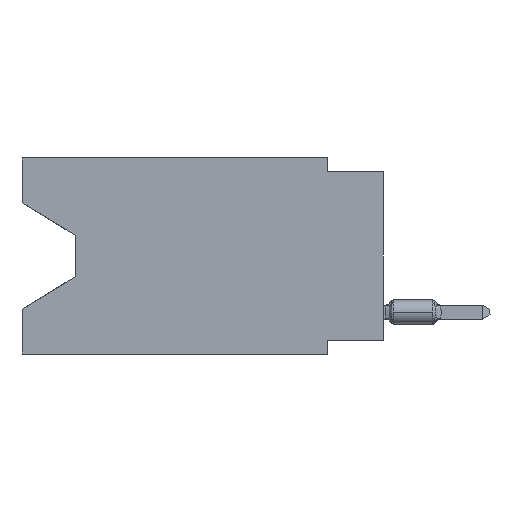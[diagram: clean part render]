
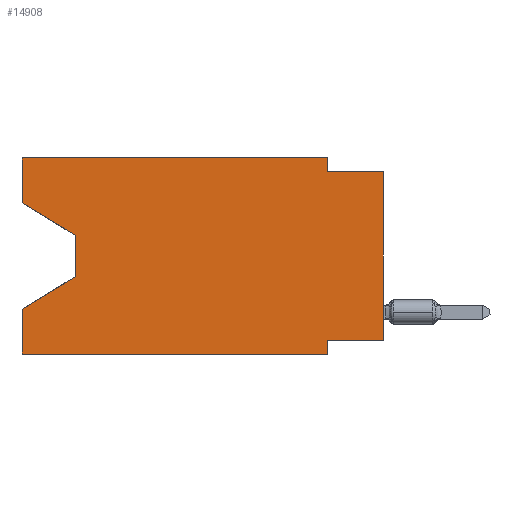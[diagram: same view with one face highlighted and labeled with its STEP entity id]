
A CAD part, left-side view. The second image highlights one B-rep face of the part: STEP entity #14908.
In plain terms, the highlighted planar face has unit normal (-1, 0, 0).
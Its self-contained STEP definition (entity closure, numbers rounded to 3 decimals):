
#5 = CARTESIAN_POINT ( 'NONE',  ( 0., 16.383, -8.89 ) ) ;
#255 = DIRECTION ( 'NONE',  ( 0., -1., 0. ) ) ;
#347 = VERTEX_POINT ( 'NONE', #15128 ) ;
#848 = LINE ( 'NONE', #18604, #24250 ) ;
#1271 = DIRECTION ( 'NONE',  ( 0., -1., 0. ) ) ;
#1398 = CARTESIAN_POINT ( 'NONE',  ( 0., 16.383, 0. ) ) ;
#1556 = CARTESIAN_POINT ( 'NONE',  ( 0., 13.97, -5.385 ) ) ;
#2352 = VERTEX_POINT ( 'NONE', #7971 ) ;
#2392 = VECTOR ( 'NONE', #1271, 1000. ) ;
#2432 = ORIENTED_EDGE ( 'NONE', *, *, #12009, .F. ) ;
#2817 = DIRECTION ( 'NONE',  ( 0., 1., 0. ) ) ;
#3191 = CARTESIAN_POINT ( 'NONE',  ( 0., 13.97, -3.505 ) ) ;
#3424 = EDGE_CURVE ( 'NONE', #2352, #17544, #19180, .T. ) ;
#3580 = VECTOR ( 'NONE', #3627, 1000. ) ;
#3627 = DIRECTION ( 'NONE',  ( 0., 0., 1. ) ) ;
#3709 = CARTESIAN_POINT ( 'NONE',  ( 0., 16.383, -2.038 ) ) ;
#4461 = VECTOR ( 'NONE', #10845, 1000. ) ;
#4632 = ORIENTED_EDGE ( 'NONE', *, *, #6374, .F. ) ;
#4938 = EDGE_CURVE ( 'NONE', #18866, #10406, #14768, .T. ) ;
#4984 = DIRECTION ( 'NONE',  ( 0., 0., 1. ) ) ;
#5467 = DIRECTION ( 'NONE',  ( 0., 0., -1. ) ) ;
#5589 = LINE ( 'NONE', #13303, #7961 ) ;
#5597 = VECTOR ( 'NONE', #24941, 1000. ) ;
#5640 = CARTESIAN_POINT ( 'NONE',  ( 0., 2.54, -8.89 ) ) ;
#5714 = DIRECTION ( 'NONE',  ( 0., -0.855, -0.519 ) ) ;
#5738 = CARTESIAN_POINT ( 'NONE',  ( 0., 16.383, 0. ) ) ;
#6042 = VERTEX_POINT ( 'NONE', #5640 ) ;
#6374 = EDGE_CURVE ( 'NONE', #17475, #347, #20489, .T. ) ;
#7307 = DIRECTION ( 'NONE',  ( 0., 0., -1. ) ) ;
#7353 = CARTESIAN_POINT ( 'NONE',  ( 0., 0., -0.635 ) ) ;
#7961 = VECTOR ( 'NONE', #5467, 1000. ) ;
#7971 = CARTESIAN_POINT ( 'NONE',  ( 0., 13.97, -5.385 ) ) ;
#8247 = VECTOR ( 'NONE', #255, 1000. ) ;
#8417 = FACE_OUTER_BOUND ( 'NONE', #22489, .T. ) ;
#8743 = CARTESIAN_POINT ( 'NONE',  ( 0., 13.97, -3.505 ) ) ;
#8981 = CARTESIAN_POINT ( 'NONE',  ( 0., 2.54, 0. ) ) ;
#9405 = EDGE_CURVE ( 'NONE', #24299, #10406, #15676, .T. ) ;
#9772 = ORIENTED_EDGE ( 'NONE', *, *, #4938, .F. ) ;
#10406 = VERTEX_POINT ( 'NONE', #7353 ) ;
#10473 = DIRECTION ( 'NONE',  ( 0., 0., -1. ) ) ;
#10730 = EDGE_CURVE ( 'NONE', #24299, #14086, #20434, .T. ) ;
#10845 = DIRECTION ( 'NONE',  ( 0., -1., 0. ) ) ;
#11954 = ORIENTED_EDGE ( 'NONE', *, *, #15281, .T. ) ;
#12009 = EDGE_CURVE ( 'NONE', #20213, #17544, #19030, .T. ) ;
#12262 = EDGE_CURVE ( 'NONE', #25340, #17475, #848, .T. ) ;
#12410 = VECTOR ( 'NONE', #25116, 1000. ) ;
#13276 = ORIENTED_EDGE ( 'NONE', *, *, #3424, .T. ) ;
#13303 = CARTESIAN_POINT ( 'NONE',  ( 0., 2.54, -8.89 ) ) ;
#13310 = VECTOR ( 'NONE', #5714, 1000. ) ;
#13683 = EDGE_CURVE ( 'NONE', #15964, #2352, #17064, .T. ) ;
#14086 = VERTEX_POINT ( 'NONE', #15706 ) ;
#14324 = PLANE ( 'NONE',  #23954 ) ;
#14700 = ORIENTED_EDGE ( 'NONE', *, *, #12262, .F. ) ;
#14768 = LINE ( 'NONE', #19029, #2392 ) ;
#14908 = ADVANCED_FACE ( 'NONE', ( #8417 ), #14324, .F. ) ;
#15128 = CARTESIAN_POINT ( 'NONE',  ( 0., 2.54, 0. ) ) ;
#15230 = EDGE_CURVE ( 'NONE', #14086, #6042, #5589, .T. ) ;
#15268 = LINE ( 'NONE', #8981, #5597 ) ;
#15281 = EDGE_CURVE ( 'NONE', #25340, #15964, #15470, .T. ) ;
#15470 = LINE ( 'NONE', #23341, #13310 ) ;
#15533 = DIRECTION ( 'NONE',  ( 0., 0., 1. ) ) ;
#15607 = VECTOR ( 'NONE', #15533, 1000. ) ;
#15676 = LINE ( 'NONE', #19803, #3580 ) ;
#15706 = CARTESIAN_POINT ( 'NONE',  ( 0., 2.54, -8.255 ) ) ;
#15964 = VERTEX_POINT ( 'NONE', #8743 ) ;
#16477 = VECTOR ( 'NONE', #2817, 1000. ) ;
#16571 = ORIENTED_EDGE ( 'NONE', *, *, #18057, .F. ) ;
#17064 = LINE ( 'NONE', #3191, #24024 ) ;
#17475 = VERTEX_POINT ( 'NONE', #5738 ) ;
#17544 = VERTEX_POINT ( 'NONE', #21934 ) ;
#17572 = ORIENTED_EDGE ( 'NONE', *, *, #13683, .T. ) ;
#18057 = EDGE_CURVE ( 'NONE', #347, #18866, #15268, .T. ) ;
#18187 = DIRECTION ( 'NONE',  ( 1., 0., 0. ) ) ;
#18604 = CARTESIAN_POINT ( 'NONE',  ( 0., 16.383, 0. ) ) ;
#18866 = VERTEX_POINT ( 'NONE', #20488 ) ;
#19029 = CARTESIAN_POINT ( 'NONE',  ( 0., 0., -0.635 ) ) ;
#19030 = LINE ( 'NONE', #1398, #15607 ) ;
#19180 = LINE ( 'NONE', #1556, #12410 ) ;
#19466 = LINE ( 'NONE', #25264, #8247 ) ;
#19803 = CARTESIAN_POINT ( 'NONE',  ( 0., 0., 0. ) ) ;
#20213 = VERTEX_POINT ( 'NONE', #5 ) ;
#20434 = LINE ( 'NONE', #20698, #16477 ) ;
#20488 = CARTESIAN_POINT ( 'NONE',  ( 0., 2.54, -0.635 ) ) ;
#20489 = LINE ( 'NONE', #20753, #4461 ) ;
#20698 = CARTESIAN_POINT ( 'NONE',  ( 0., 0., -8.255 ) ) ;
#20753 = CARTESIAN_POINT ( 'NONE',  ( 0., 16.383, 0. ) ) ;
#20826 = CARTESIAN_POINT ( 'NONE',  ( 0., 0., -8.255 ) ) ;
#21405 = EDGE_CURVE ( 'NONE', #20213, #6042, #19466, .T. ) ;
#21700 = ORIENTED_EDGE ( 'NONE', *, *, #9405, .T. ) ;
#21934 = CARTESIAN_POINT ( 'NONE',  ( 0., 16.383, -6.852 ) ) ;
#22489 = EDGE_LOOP ( 'NONE', ( #11954, #17572, #13276, #2432, #24428, #23222, #23672, #21700, #9772, #16571, #4632, #14700 ) ) ;
#23222 = ORIENTED_EDGE ( 'NONE', *, *, #15230, .F. ) ;
#23341 = CARTESIAN_POINT ( 'NONE',  ( 0., 16.383, -2.038 ) ) ;
#23672 = ORIENTED_EDGE ( 'NONE', *, *, #10730, .F. ) ;
#23954 = AXIS2_PLACEMENT_3D ( 'NONE', #24113, #18187, #10473 ) ;
#24024 = VECTOR ( 'NONE', #7307, 1000. ) ;
#24113 = CARTESIAN_POINT ( 'NONE',  ( 0., 16.383, 0. ) ) ;
#24250 = VECTOR ( 'NONE', #4984, 1000. ) ;
#24299 = VERTEX_POINT ( 'NONE', #20826 ) ;
#24428 = ORIENTED_EDGE ( 'NONE', *, *, #21405, .T. ) ;
#24941 = DIRECTION ( 'NONE',  ( 0., 0., -1. ) ) ;
#25116 = DIRECTION ( 'NONE',  ( 0., 0.855, -0.519 ) ) ;
#25264 = CARTESIAN_POINT ( 'NONE',  ( 0., 16.383, -8.89 ) ) ;
#25340 = VERTEX_POINT ( 'NONE', #3709 ) ;
